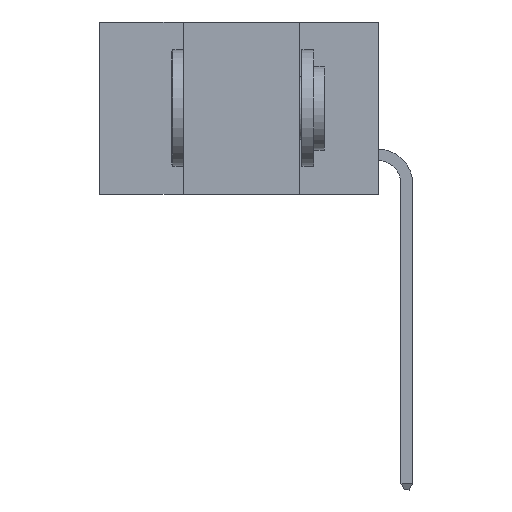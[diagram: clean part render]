
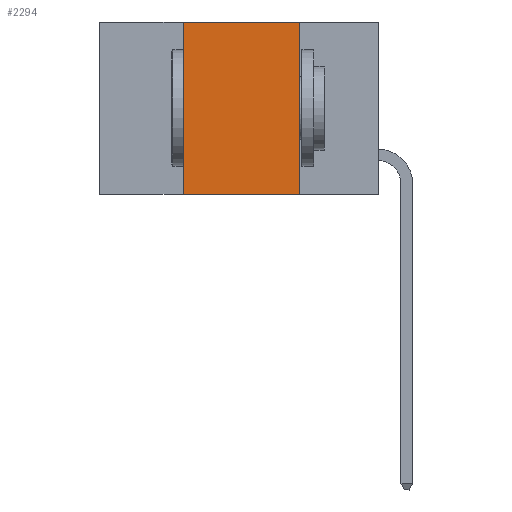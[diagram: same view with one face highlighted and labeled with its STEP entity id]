
A CAD part, left-side view. The second image highlights one B-rep face of the part: STEP entity #2294.
In plain terms, the highlighted planar face has unit normal (-1, 0, 0).
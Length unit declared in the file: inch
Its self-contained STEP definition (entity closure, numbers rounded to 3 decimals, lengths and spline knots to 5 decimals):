
#159 = LINE ( 'NONE', #4386, #9903 ) ;
#740 = EDGE_CURVE ( 'NONE', #3761, #4183, #159, .T. ) ;
#767 = VECTOR ( 'NONE', #5612, 39.37008 ) ;
#959 = CARTESIAN_POINT ( 'NONE',  ( 0., 0.6, -0.37 ) ) ;
#2058 = ORIENTED_EDGE ( 'NONE', *, *, #4864, .F. ) ;
#2218 = ORIENTED_EDGE ( 'NONE', *, *, #3515, .T. ) ;
#2294 = ADVANCED_FACE ( 'NONE', ( #5087 ), #12394, .F. ) ;
#2300 = EDGE_CURVE ( 'NONE', #10696, #10165, #2454, .T. ) ;
#2454 = LINE ( 'NONE', #7799, #4795 ) ;
#3515 = EDGE_CURVE ( 'NONE', #10696, #4183, #11467, .T. ) ;
#3642 = ORIENTED_EDGE ( 'NONE', *, *, #2300, .F. ) ;
#3699 = CARTESIAN_POINT ( 'NONE',  ( 0., 0.42, -0.37 ) ) ;
#3761 = VERTEX_POINT ( 'NONE', #4987 ) ;
#4039 = CARTESIAN_POINT ( 'NONE',  ( 0., 0.17, -0.37 ) ) ;
#4068 = EDGE_LOOP ( 'NONE', ( #11579, #2058, #3642, #2218 ) ) ;
#4183 = VERTEX_POINT ( 'NONE', #4039 ) ;
#4356 = DIRECTION ( 'NONE',  ( 0., 0., -1. ) ) ;
#4386 = CARTESIAN_POINT ( 'NONE',  ( 0., 0.17, 0. ) ) ;
#4394 = AXIS2_PLACEMENT_3D ( 'NONE', #7392, #7374, #5748 ) ;
#4485 = CARTESIAN_POINT ( 'NONE',  ( 0., 0.6, 0. ) ) ;
#4795 = VECTOR ( 'NONE', #12333, 39.37008 ) ;
#4864 = EDGE_CURVE ( 'NONE', #10165, #3761, #8582, .T. ) ;
#4987 = CARTESIAN_POINT ( 'NONE',  ( 0., 0.17, 0. ) ) ;
#5087 = FACE_OUTER_BOUND ( 'NONE', #4068, .T. ) ;
#5612 = DIRECTION ( 'NONE',  ( 0., -1., 0. ) ) ;
#5748 = DIRECTION ( 'NONE',  ( 0., 0., -1. ) ) ;
#6359 = DIRECTION ( 'NONE',  ( 0., -1., 0. ) ) ;
#7374 = DIRECTION ( 'NONE',  ( 1., 0., 0. ) ) ;
#7392 = CARTESIAN_POINT ( 'NONE',  ( 0., 0.6, 0. ) ) ;
#7528 = CARTESIAN_POINT ( 'NONE',  ( 0., 0.42, 0. ) ) ;
#7799 = CARTESIAN_POINT ( 'NONE',  ( 0., 0.42, 0. ) ) ;
#8582 = LINE ( 'NONE', #4485, #767 ) ;
#9039 = VECTOR ( 'NONE', #6359, 39.37008 ) ;
#9903 = VECTOR ( 'NONE', #4356, 39.37008 ) ;
#10165 = VERTEX_POINT ( 'NONE', #7528 ) ;
#10696 = VERTEX_POINT ( 'NONE', #3699 ) ;
#11467 = LINE ( 'NONE', #959, #9039 ) ;
#11579 = ORIENTED_EDGE ( 'NONE', *, *, #740, .F. ) ;
#12333 = DIRECTION ( 'NONE',  ( 0., 0., 1. ) ) ;
#12394 = PLANE ( 'NONE',  #4394 ) ;
